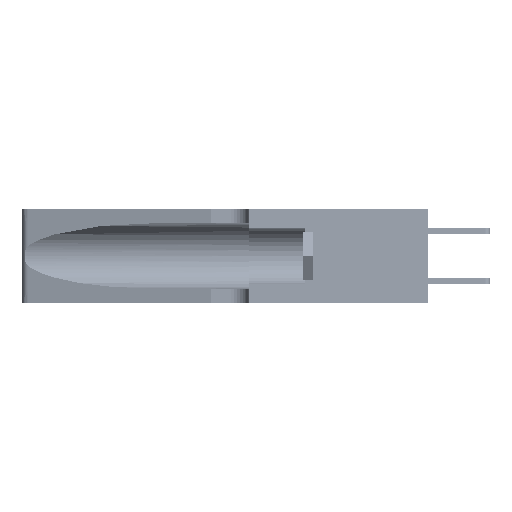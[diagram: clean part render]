
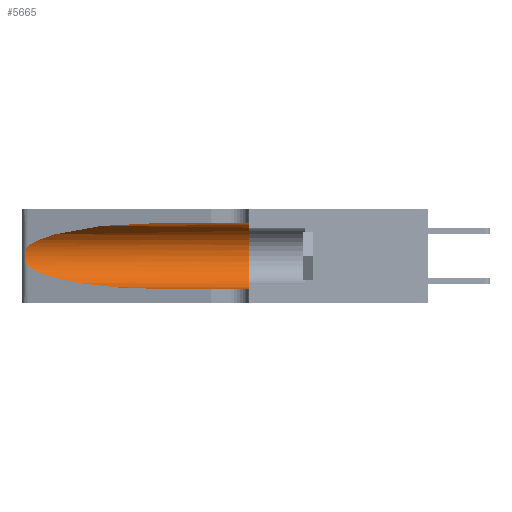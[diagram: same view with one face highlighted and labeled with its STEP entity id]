
A CAD part, left-side view. The second image highlights one B-rep face of the part: STEP entity #5665.
In plain terms, the highlighted cylindrical face has radius 3.308 mm (diameter 6.617 mm), a partial arc.
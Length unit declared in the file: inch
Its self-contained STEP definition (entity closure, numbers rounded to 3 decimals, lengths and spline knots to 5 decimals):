
#478 = CARTESIAN_POINT ( 'NONE',  ( 0.25639, 1.23186, 0.15144 ) ) ;
#1158 = CARTESIAN_POINT ( 'NONE',  ( 0.2373, 1.15595, 0.08982 ) ) ;
#2244 = VERTEX_POINT ( 'NONE', #35146 ) ;
#2950 = CARTESIAN_POINT ( 'NONE',  ( 0.1305, 0.35, 0.185 ) ) ;
#3250 = CARTESIAN_POINT ( 'NONE',  ( 0.1305, 0.72297, 0.05475 ) ) ;
#3368 = CARTESIAN_POINT ( 'NONE',  ( 0.1305, 0.72297, 0.31525 ) ) ;
#3421 = CARTESIAN_POINT ( 'NONE',  ( 0.26075, 1.23896, 0.19203 ) ) ;
#4710 = EDGE_CURVE ( 'NONE', #18294, #2244, #22993, .T. ) ;
#4723 = CARTESIAN_POINT ( 'NONE',  ( 0.18966, 0.96281, 0.05475 ) ) ;
#5665 = ADVANCED_FACE ( 'NONE', ( #37812 ), #27352, .F. ) ;
#5760 = CARTESIAN_POINT ( 'NONE',  ( 0.1305, 0.35, 0.31525 ) ) ;
#6724 = CARTESIAN_POINT ( 'NONE',  ( 0.1305, 1.61858, 0.185 ) ) ;
#6920 = CARTESIAN_POINT ( 'NONE',  ( 0.18966, 0.96281, 0.31525 ) ) ;
#8012 = CARTESIAN_POINT ( 'NONE',  ( 0.26075, 1.23896, 0.178 ) ) ;
#8923 = EDGE_CURVE ( 'NONE', #2244, #42851, #24143, .T. ) ;
#9912 = ORIENTED_EDGE ( 'NONE', *, *, #4710, .T. ) ;
#10860 = DIRECTION ( 'NONE',  ( 0., -1., 0. ) ) ;
#12325 = VERTEX_POINT ( 'NONE', #16339 ) ;
#13265 = CARTESIAN_POINT ( 'NONE',  ( 0.25487, 1.22718, 0.22369 ) ) ;
#14018 = CARTESIAN_POINT ( 'NONE',  ( 0.1305, 0.35, 0.05475 ) ) ;
#14365 = CARTESIAN_POINT ( 'NONE',  ( 0.25787, 1.23484, 0.2124 ) ) ;
#14673 = CARTESIAN_POINT ( 'NONE',  ( 0.25487, 1.22718, 0.14631 ) ) ;
#15042 =( BOUNDED_CURVE ( )  B_SPLINE_CURVE ( 3, ( #3368, #6920, #31528, #13265 ),
 .UNSPECIFIED., .F., .T. ) 
 B_SPLINE_CURVE_WITH_KNOTS ( ( 4, 4 ),
 ( 1.5708, 2.84003 ),
 .UNSPECIFIED. ) 
 CURVE ( )  GEOMETRIC_REPRESENTATION_ITEM ( )  RATIONAL_B_SPLINE_CURVE ( ( 1., 0.87, 0.87, 1. ) ) 
 REPRESENTATION_ITEM ( '' )  );
#16339 = CARTESIAN_POINT ( 'NONE',  ( 0.1305, 0.72297, 0.31525 ) ) ;
#17016 = ORIENTED_EDGE ( 'NONE', *, *, #45036, .F. ) ;
#17776 = CARTESIAN_POINT ( 'NONE',  ( 0.25854, 1.2359, 0.20912 ) ) ;
#17929 = LINE ( 'NONE', #45300, #31651 ) ;
#18294 = VERTEX_POINT ( 'NONE', #28446 ) ;
#18652 = LINE ( 'NONE', #34063, #36248 ) ;
#20752 = EDGE_CURVE ( 'NONE', #12325, #36823, #18652, .T. ) ;
#22993 = B_SPLINE_CURVE_WITH_KNOTS ( 'NONE', 3,
 ( #31428, #34974, #24550, #14365, #17776, #38990, #3421, #8012, #39441, #29138, #32481, #478, #28995, #14673 ),
 .UNSPECIFIED., .F., .F.,
 ( 4, 2, 2, 2, 2, 2, 4 ),
 ( 0., 0.00027, 0.00053, 0.00107, 0.0016, 0.00187, 0.00214 ),
 .UNSPECIFIED. ) ;
#24143 =( BOUNDED_CURVE ( )  B_SPLINE_CURVE ( 3, ( #33030, #1158, #4723, #32882 ),
 .UNSPECIFIED., .F., .T. ) 
 B_SPLINE_CURVE_WITH_KNOTS ( ( 4, 4 ),
 ( 3.44316, 4.71239 ),
 .UNSPECIFIED. ) 
 CURVE ( )  GEOMETRIC_REPRESENTATION_ITEM ( )  RATIONAL_B_SPLINE_CURVE ( ( 1., 0.87, 0.87, 1. ) ) 
 REPRESENTATION_ITEM ( '' )  );
#24550 = CARTESIAN_POINT ( 'NONE',  ( 0.25639, 1.23184, 0.21858 ) ) ;
#25377 = ORIENTED_EDGE ( 'NONE', *, *, #20752, .F. ) ;
#27176 = DIRECTION ( 'NONE',  ( 0., -1., 0. ) ) ;
#27352 = CYLINDRICAL_SURFACE ( 'NONE', #38151, 0.13025 ) ;
#27855 = ORIENTED_EDGE ( 'NONE', *, *, #41992, .T. ) ;
#28446 = CARTESIAN_POINT ( 'NONE',  ( 0.25487, 1.22718, 0.22369 ) ) ;
#28995 = CARTESIAN_POINT ( 'NONE',  ( 0.25555, 1.22993, 0.14849 ) ) ;
#29138 = CARTESIAN_POINT ( 'NONE',  ( 0.25856, 1.23593, 0.16098 ) ) ;
#29973 = AXIS2_PLACEMENT_3D ( 'NONE', #2950, #34792, #34959 ) ;
#31336 = DIRECTION ( 'NONE',  ( 0., -1., 0. ) ) ;
#31428 = CARTESIAN_POINT ( 'NONE',  ( 0.25487, 1.22718, 0.22369 ) ) ;
#31528 = CARTESIAN_POINT ( 'NONE',  ( 0.2373, 1.15595, 0.28018 ) ) ;
#31651 = VECTOR ( 'NONE', #10860, 39.37008 ) ;
#32049 = VERTEX_POINT ( 'NONE', #14018 ) ;
#32481 = CARTESIAN_POINT ( 'NONE',  ( 0.25789, 1.23486, 0.15765 ) ) ;
#32632 = EDGE_LOOP ( 'NONE', ( #27855, #9912, #36438, #35792, #17016, #25377 ) ) ;
#32882 = CARTESIAN_POINT ( 'NONE',  ( 0.1305, 0.72297, 0.05475 ) ) ;
#33030 = CARTESIAN_POINT ( 'NONE',  ( 0.25487, 1.22718, 0.14631 ) ) ;
#34063 = CARTESIAN_POINT ( 'NONE',  ( 0.1305, 1.61858, 0.31525 ) ) ;
#34792 = DIRECTION ( 'NONE',  ( 0., 1., 0. ) ) ;
#34959 = DIRECTION ( 'NONE',  ( 0., 0., 1. ) ) ;
#34974 = CARTESIAN_POINT ( 'NONE',  ( 0.25555, 1.22994, 0.2215 ) ) ;
#35146 = CARTESIAN_POINT ( 'NONE',  ( 0.25487, 1.22718, 0.14631 ) ) ;
#35792 = ORIENTED_EDGE ( 'NONE', *, *, #44538, .T. ) ;
#36248 = VECTOR ( 'NONE', #27176, 39.37008 ) ;
#36438 = ORIENTED_EDGE ( 'NONE', *, *, #8923, .T. ) ;
#36823 = VERTEX_POINT ( 'NONE', #5760 ) ;
#37812 = FACE_OUTER_BOUND ( 'NONE', #32632, .T. ) ;
#38129 = DIRECTION ( 'NONE',  ( 0., 0., -1. ) ) ;
#38151 = AXIS2_PLACEMENT_3D ( 'NONE', #6724, #31336, #38129 ) ;
#38990 = CARTESIAN_POINT ( 'NONE',  ( 0.26018, 1.23835, 0.19895 ) ) ;
#39441 = CARTESIAN_POINT ( 'NONE',  ( 0.26017, 1.23833, 0.17102 ) ) ;
#41992 = EDGE_CURVE ( 'NONE', #12325, #18294, #15042, .T. ) ;
#42851 = VERTEX_POINT ( 'NONE', #3250 ) ;
#44538 = EDGE_CURVE ( 'NONE', #42851, #32049, #17929, .T. ) ;
#45036 = EDGE_CURVE ( 'NONE', #36823, #32049, #45391, .T. ) ;
#45300 = CARTESIAN_POINT ( 'NONE',  ( 0.1305, 1.61858, 0.05475 ) ) ;
#45391 = CIRCLE ( 'NONE', #29973, 0.13025 ) ;
